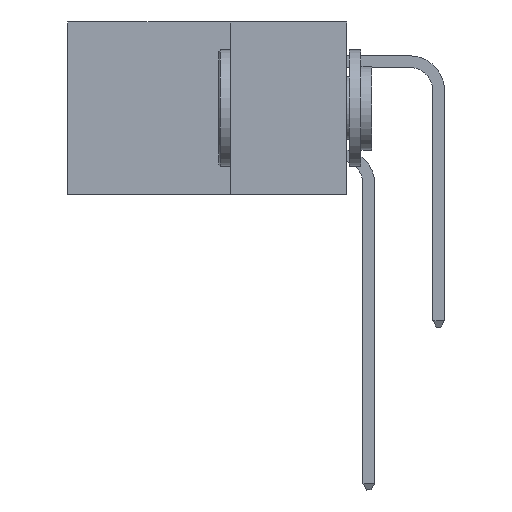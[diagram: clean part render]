
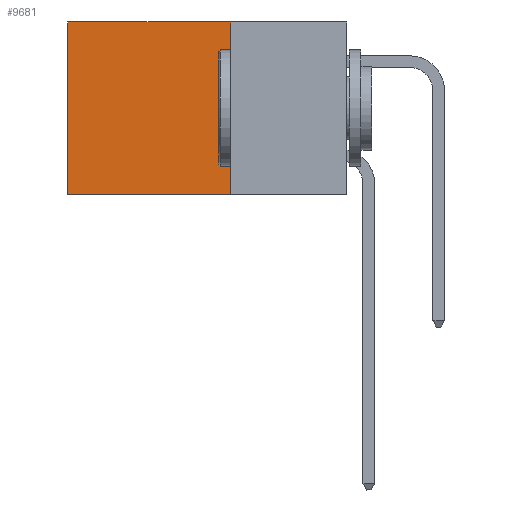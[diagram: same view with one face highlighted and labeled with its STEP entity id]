
A CAD part, left-side view. The second image highlights one B-rep face of the part: STEP entity #9681.
In plain terms, the highlighted planar face has unit normal (-1, 0, 0).
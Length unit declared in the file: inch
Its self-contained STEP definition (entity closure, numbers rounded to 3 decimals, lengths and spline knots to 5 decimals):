
#209 = EDGE_CURVE ( 'NONE', #33013, #15074, #10359, .T. ) ;
#351 = CARTESIAN_POINT ( 'NONE',  ( 0.2875, 0.25, 0. ) ) ;
#445 = CARTESIAN_POINT ( 'NONE',  ( 0.2875, 0.6, 0. ) ) ;
#2273 = DIRECTION ( 'NONE',  ( 0., 0., -1. ) ) ;
#3098 = LINE ( 'NONE', #23523, #37946 ) ;
#3265 = CARTESIAN_POINT ( 'NONE',  ( 0.2875, 0.25, 0. ) ) ;
#9681 = ADVANCED_FACE ( 'NONE', ( #39194 ), #28425, .F. ) ;
#10339 = VECTOR ( 'NONE', #10571, 39.37008 ) ;
#10359 = LINE ( 'NONE', #30853, #17053 ) ;
#10571 = DIRECTION ( 'NONE',  ( 0., 1., 0. ) ) ;
#13754 = EDGE_CURVE ( 'NONE', #17331, #20589, #19075, .T. ) ;
#14909 = CARTESIAN_POINT ( 'NONE',  ( 0.2875, 0.6, 0. ) ) ;
#15074 = VERTEX_POINT ( 'NONE', #41470 ) ;
#17053 = VECTOR ( 'NONE', #27595, 39.37008 ) ;
#17331 = VERTEX_POINT ( 'NONE', #3265 ) ;
#18832 = ORIENTED_EDGE ( 'NONE', *, *, #33966, .T. ) ;
#19075 = LINE ( 'NONE', #351, #10339 ) ;
#20589 = VERTEX_POINT ( 'NONE', #445 ) ;
#21200 = EDGE_CURVE ( 'NONE', #17331, #33013, #3098, .T. ) ;
#21677 = ORIENTED_EDGE ( 'NONE', *, *, #13754, .T. ) ;
#21915 = DIRECTION ( 'NONE',  ( 1., 0., 0. ) ) ;
#22055 = CARTESIAN_POINT ( 'NONE',  ( 0.2875, 0.25, 0. ) ) ;
#23523 = CARTESIAN_POINT ( 'NONE',  ( 0.2875, 0.25, 0. ) ) ;
#26632 = DIRECTION ( 'NONE',  ( 0., 0., -1. ) ) ;
#27077 = AXIS2_PLACEMENT_3D ( 'NONE', #22055, #21915, #2273 ) ;
#27595 = DIRECTION ( 'NONE',  ( 0., 1., 0. ) ) ;
#27989 = DIRECTION ( 'NONE',  ( 0., 0., -1. ) ) ;
#28174 = VECTOR ( 'NONE', #27989, 39.37008 ) ;
#28425 = PLANE ( 'NONE',  #27077 ) ;
#29177 = LINE ( 'NONE', #14909, #28174 ) ;
#30853 = CARTESIAN_POINT ( 'NONE',  ( 0.2875, 0.25, -0.37 ) ) ;
#33013 = VERTEX_POINT ( 'NONE', #35756 ) ;
#33368 = ORIENTED_EDGE ( 'NONE', *, *, #21200, .F. ) ;
#33846 = EDGE_LOOP ( 'NONE', ( #18832, #35578, #33368, #21677 ) ) ;
#33966 = EDGE_CURVE ( 'NONE', #20589, #15074, #29177, .T. ) ;
#35578 = ORIENTED_EDGE ( 'NONE', *, *, #209, .F. ) ;
#35756 = CARTESIAN_POINT ( 'NONE',  ( 0.2875, 0.25, -0.37 ) ) ;
#37946 = VECTOR ( 'NONE', #26632, 39.37008 ) ;
#39194 = FACE_OUTER_BOUND ( 'NONE', #33846, .T. ) ;
#41470 = CARTESIAN_POINT ( 'NONE',  ( 0.2875, 0.6, -0.37 ) ) ;
